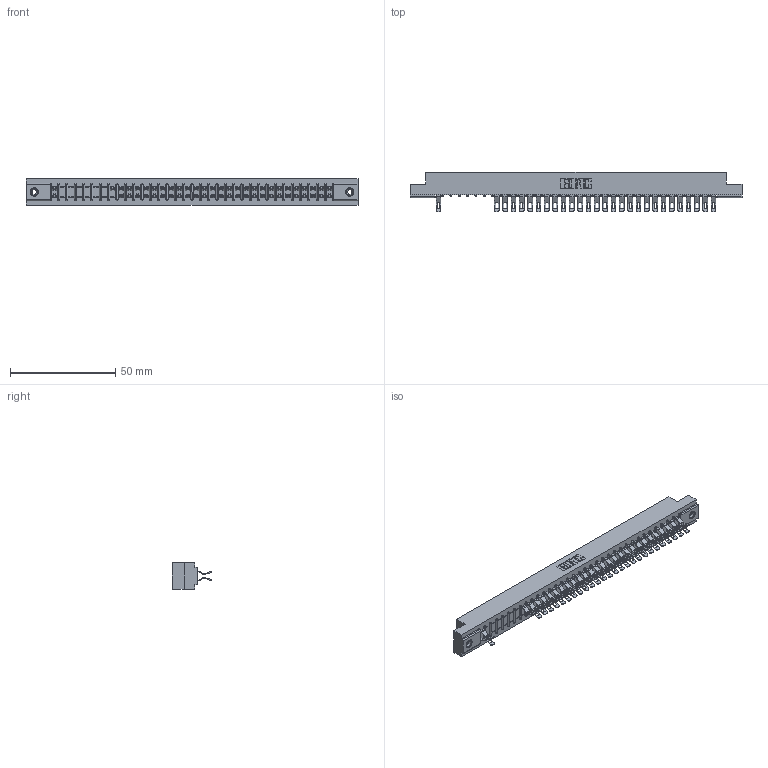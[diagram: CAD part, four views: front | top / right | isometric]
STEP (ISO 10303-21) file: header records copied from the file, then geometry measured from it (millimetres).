
FILE_DESCRIPTION (( 'STEP AP203' ), '1' );
FILE_NAME ('307-068-555-208.STEP', '2018-08-06T12:11:42', ( '' ), ( '' ), 'SwSTEP 2.0', 'SolidWorks 2016', '' );
FILE_SCHEMA (( 'CONFIG_CONTROL_DESIGN' ));
Length unit declared in the file: inch
Products named in the file (4): 307 Part_.156 Dia Mounting Holes; 307-290-001_555; 345-250-001_345-250-003-102; 307-068-555-208
Assembly tree (58 placements, depth 2):
  307-068-555-208
    307 Part_.156 Dia Mounting Holes
    307-290-001_555  x55
    345-250-001_345-250-003-102  x2
Bounding box: 157.73 x 18.75 x 12.7 mm (x, y, z)
Volume: 16705.5 mm3; surface area: 20103.5 mm2
Topology: 58 solids, 58 shells, 3698 faces, 10830 edges, 7044 vertices
Faces by surface type: plane 2050, cylinder 1562, sphere 70, cone 12, torus 4
Entity records: 32528 total; most frequent: CARTESIAN_POINT 5368, ORIENTED_EDGE 5328, DIRECTION 5264, EDGE_CURVE 2664, VECTOR 2028, LINE 2028, VERTEX_POINT 1722, AXIS2_PLACEMENT_3D 1618
